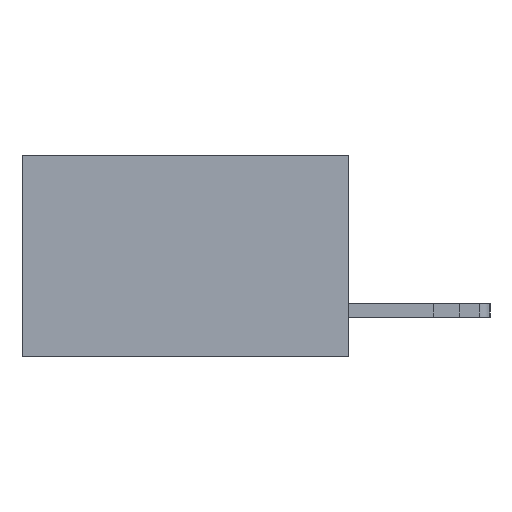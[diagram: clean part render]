
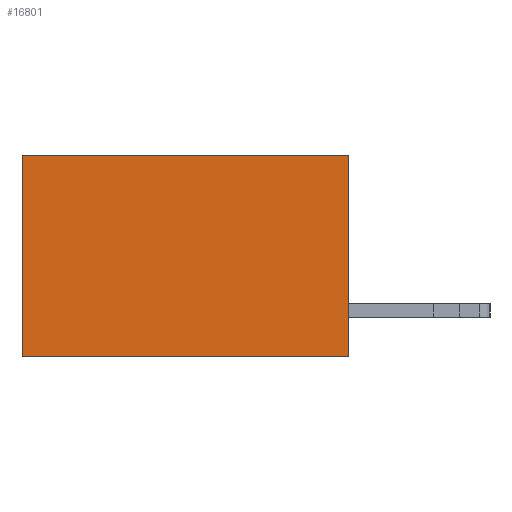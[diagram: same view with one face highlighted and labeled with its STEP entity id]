
A CAD part, left-side view. The second image highlights one B-rep face of the part: STEP entity #16801.
In plain terms, the highlighted planar face has unit normal (-1, 0, 0).
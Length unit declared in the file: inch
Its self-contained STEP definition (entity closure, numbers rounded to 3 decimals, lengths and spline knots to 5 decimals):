
#295 = EDGE_LOOP ( 'NONE', ( #4139, #4256, #3994, #2312 ) ) ;
#419 = DIRECTION ( 'NONE',  ( 0., 0., -1. ) ) ;
#450 = LINE ( 'NONE', #5156, #3467 ) ;
#565 = EDGE_CURVE ( 'NONE', #14317, #8794, #15128, .T. ) ;
#705 = EDGE_CURVE ( 'NONE', #13831, #9254, #15772, .T. ) ;
#2312 = ORIENTED_EDGE ( 'NONE', *, *, #9170, .T. ) ;
#2515 = VECTOR ( 'NONE', #13386, 39.37008 ) ;
#2705 = CARTESIAN_POINT ( 'NONE',  ( 0.298, 0., 0. ) ) ;
#3329 = CARTESIAN_POINT ( 'NONE',  ( 0.298, 0., -0.37 ) ) ;
#3467 = VECTOR ( 'NONE', #10505, 39.37008 ) ;
#3994 = ORIENTED_EDGE ( 'NONE', *, *, #705, .F. ) ;
#4139 = ORIENTED_EDGE ( 'NONE', *, *, #565, .T. ) ;
#4207 = DIRECTION ( 'NONE',  ( 0., 0., -1. ) ) ;
#4256 = ORIENTED_EDGE ( 'NONE', *, *, #14983, .F. ) ;
#4508 = CARTESIAN_POINT ( 'NONE',  ( 0.298, 0.6, 0. ) ) ;
#5156 = CARTESIAN_POINT ( 'NONE',  ( 0.298, 0., 0. ) ) ;
#6090 = FACE_OUTER_BOUND ( 'NONE', #295, .T. ) ;
#6391 = LINE ( 'NONE', #3329, #2515 ) ;
#6571 = CARTESIAN_POINT ( 'NONE',  ( 0.298, 0.6, 0. ) ) ;
#6999 = PLANE ( 'NONE',  #14746 ) ;
#8794 = VERTEX_POINT ( 'NONE', #15913 ) ;
#9170 = EDGE_CURVE ( 'NONE', #13831, #14317, #450, .T. ) ;
#9254 = VERTEX_POINT ( 'NONE', #10610 ) ;
#10505 = DIRECTION ( 'NONE',  ( 0., 1., 0. ) ) ;
#10610 = CARTESIAN_POINT ( 'NONE',  ( 0.298, 0., -0.37 ) ) ;
#11246 = CARTESIAN_POINT ( 'NONE',  ( 0.298, 0., 0. ) ) ;
#12781 = DIRECTION ( 'NONE',  ( 0., 0., -1. ) ) ;
#12791 = DIRECTION ( 'NONE',  ( 1., 0., 0. ) ) ;
#13386 = DIRECTION ( 'NONE',  ( 0., 1., 0. ) ) ;
#13831 = VERTEX_POINT ( 'NONE', #16303 ) ;
#14317 = VERTEX_POINT ( 'NONE', #4508 ) ;
#14680 = VECTOR ( 'NONE', #12781, 39.37008 ) ;
#14746 = AXIS2_PLACEMENT_3D ( 'NONE', #2705, #12791, #4207 ) ;
#14983 = EDGE_CURVE ( 'NONE', #9254, #8794, #6391, .T. ) ;
#15128 = LINE ( 'NONE', #6571, #14680 ) ;
#15772 = LINE ( 'NONE', #11246, #16202 ) ;
#15913 = CARTESIAN_POINT ( 'NONE',  ( 0.298, 0.6, -0.37 ) ) ;
#16202 = VECTOR ( 'NONE', #419, 39.37008 ) ;
#16303 = CARTESIAN_POINT ( 'NONE',  ( 0.298, 0., 0. ) ) ;
#16801 = ADVANCED_FACE ( 'NONE', ( #6090 ), #6999, .F. ) ;
